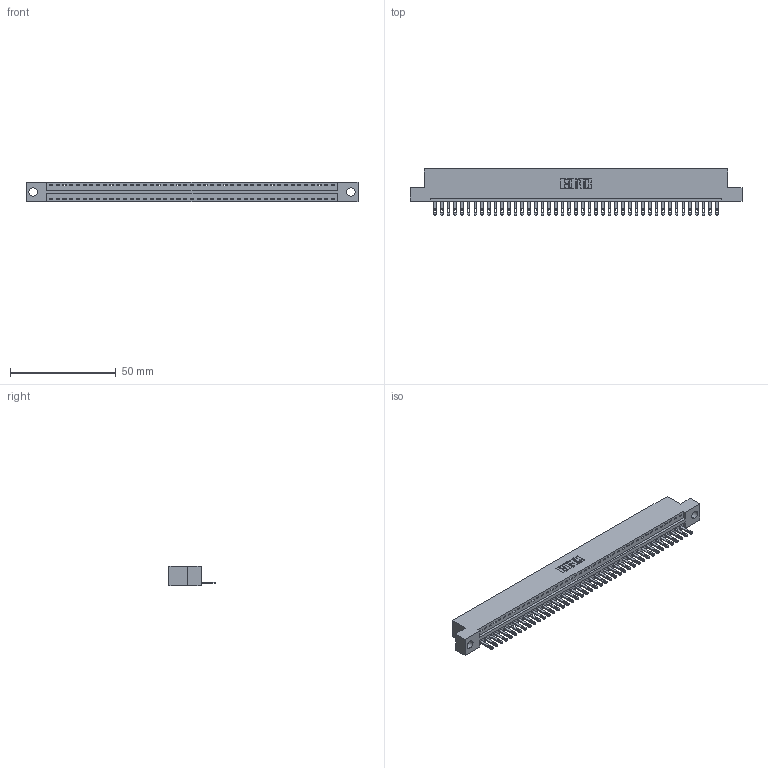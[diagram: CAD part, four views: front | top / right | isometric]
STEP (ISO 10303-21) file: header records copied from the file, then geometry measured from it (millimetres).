
FILE_DESCRIPTION (( 'STEP AP203' ), '1' );
FILE_NAME ('896-043-500-104.STEP', '2021-07-27T21:48:52', ( '' ), ( '' ), 'SwSTEP 2.0', 'SolidWorks 2020', '' );
FILE_SCHEMA (( 'CONFIG_CONTROL_DESIGN' ));
Length unit declared in the file: inch
Products named in the file (3): 846 Part_Flush Mounting Lugs - 0.156 Dia-TH; 345-292-001_345-293-100; 896-043-500-104
Assembly tree (44 placements, depth 2):
  896-043-500-104
    846 Part_Flush Mounting Lugs - 0.156 Dia-TH
    345-292-001_345-293-100  x43
Bounding box: 157.1 x 21.84 x 9.4 mm (x, y, z)
Volume: 14983.5 mm3; surface area: 18643.4 mm2
Topology: 44 solids, 44 shells, 2444 faces, 7553 edges, 5034 vertices
Faces by surface type: plane 1538, cylinder 906
Entity records: 26485 total; most frequent: CARTESIAN_POINT 4545, ORIENTED_EDGE 4522, DIRECTION 4011, EDGE_CURVE 2261, VECTOR 1953, LINE 1953, VERTEX_POINT 1506, AXIS2_PLACEMENT_3D 1029
